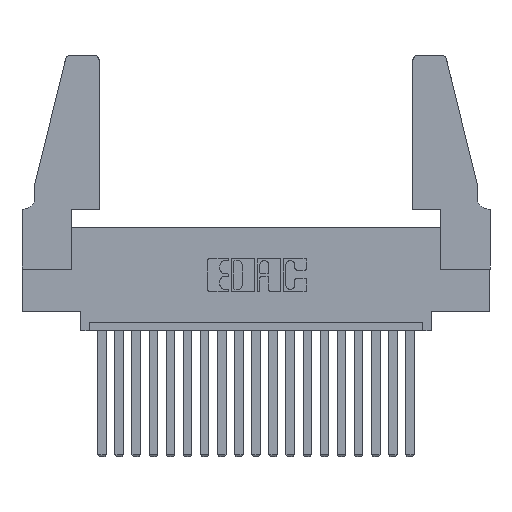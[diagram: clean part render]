
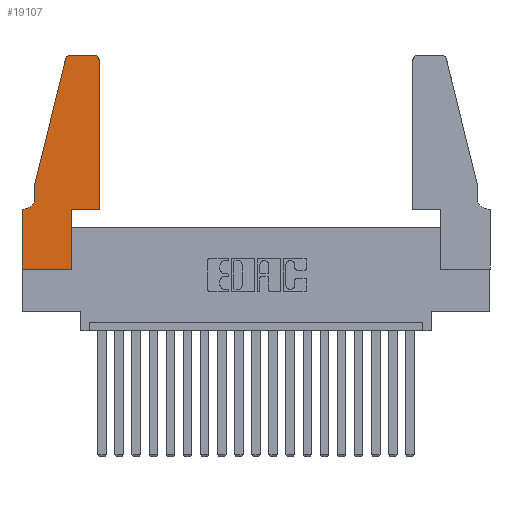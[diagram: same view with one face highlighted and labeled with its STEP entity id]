
A CAD part, top view. The second image highlights one B-rep face of the part: STEP entity #19107.
In plain terms, the highlighted planar face has unit normal (0, 0, 1).
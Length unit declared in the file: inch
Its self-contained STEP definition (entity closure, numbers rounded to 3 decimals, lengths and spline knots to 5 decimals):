
#226 = VERTEX_POINT ( 'NONE', #11601 ) ;
#607 = LINE ( 'NONE', #13470, #18976 ) ;
#1003 = FACE_OUTER_BOUND ( 'NONE', #8176, .T. ) ;
#1353 = EDGE_CURVE ( 'NONE', #18192, #9821, #18498, .T. ) ;
#1401 = EDGE_CURVE ( 'NONE', #15316, #226, #607, .T. ) ;
#1546 = CARTESIAN_POINT ( 'NONE',  ( 0.4505, 1.22, 0.37 ) ) ;
#1933 = EDGE_CURVE ( 'NONE', #9757, #9696, #8826, .T. ) ;
#2170 = DIRECTION ( 'NONE',  ( 1., 0., 0. ) ) ;
#2284 = VECTOR ( 'NONE', #16192, 39.37008 ) ;
#2330 = CARTESIAN_POINT ( 'NONE',  ( 0.4505, 0.35, 0.37 ) ) ;
#2348 = CARTESIAN_POINT ( 'NONE',  ( 0., 0., 0.37 ) ) ;
#2522 = ORIENTED_EDGE ( 'NONE', *, *, #6118, .T. ) ;
#2738 = CARTESIAN_POINT ( 'NONE',  ( 0.2605, 1.25, 0.37 ) ) ;
#2778 = LINE ( 'NONE', #10373, #2284 ) ;
#2810 = VERTEX_POINT ( 'NONE', #13792 ) ;
#2832 = DIRECTION ( 'NONE',  ( 0., -1., 0. ) ) ;
#3273 = VECTOR ( 'NONE', #3292, 39.37008 ) ;
#3292 = DIRECTION ( 'NONE',  ( 0., 1., 0. ) ) ;
#3576 = ORIENTED_EDGE ( 'NONE', *, *, #6120, .T. ) ;
#3849 = DIRECTION ( 'NONE',  ( 0., 1., 0. ) ) ;
#4026 = LINE ( 'NONE', #2738, #9886 ) ;
#4096 = ORIENTED_EDGE ( 'NONE', *, *, #1401, .T. ) ;
#4298 = DIRECTION ( 'NONE',  ( 0., 0., 1. ) ) ;
#4327 = LINE ( 'NONE', #17046, #19376 ) ;
#4695 = CARTESIAN_POINT ( 'NONE',  ( 0.2865, 0.35, 0.37 ) ) ;
#4701 = VECTOR ( 'NONE', #3849, 39.37008 ) ;
#4831 = AXIS2_PLACEMENT_3D ( 'NONE', #6130, #14998, #16462 ) ;
#5310 = ORIENTED_EDGE ( 'NONE', *, *, #9692, .T. ) ;
#5459 = DIRECTION ( 'NONE',  ( 0., -1., 0. ) ) ;
#5569 = CARTESIAN_POINT ( 'NONE',  ( 0.284, 1.25, 0.37 ) ) ;
#5737 = PLANE ( 'NONE',  #19244 ) ;
#5888 = CIRCLE ( 'NONE', #4831, 0.07 ) ;
#6118 = EDGE_CURVE ( 'NONE', #9821, #15316, #18614, .T. ) ;
#6120 = EDGE_CURVE ( 'NONE', #2810, #9757, #17877, .T. ) ;
#6130 = CARTESIAN_POINT ( 'NONE',  ( 0.0055, 0.42, 0.37 ) ) ;
#6135 = CARTESIAN_POINT ( 'NONE',  ( 0.284, 1.22, 0.37 ) ) ;
#6221 = DIRECTION ( 'NONE',  ( 1., 0., 0. ) ) ;
#6379 = VERTEX_POINT ( 'NONE', #4695 ) ;
#6643 = VERTEX_POINT ( 'NONE', #11308 ) ;
#6938 = ORIENTED_EDGE ( 'NONE', *, *, #11373, .T. ) ;
#7241 = DIRECTION ( 'NONE',  ( 1., 0., 0. ) ) ;
#7745 = VERTEX_POINT ( 'NONE', #16315 ) ;
#7936 = CARTESIAN_POINT ( 'NONE',  ( 0.2865, 0.35, 0.37 ) ) ;
#8176 = EDGE_LOOP ( 'NONE', ( #9922, #12229, #2522, #4096, #11889, #6938, #5310, #16405, #16954, #9813, #3576, #8730 ) ) ;
#8730 = ORIENTED_EDGE ( 'NONE', *, *, #1933, .T. ) ;
#8826 = CIRCLE ( 'NONE', #12240, 0.03 ) ;
#9294 = CARTESIAN_POINT ( 'NONE',  ( 0.4205, 1.22, 0.37 ) ) ;
#9692 = EDGE_CURVE ( 'NONE', #9926, #6643, #11031, .T. ) ;
#9696 = VERTEX_POINT ( 'NONE', #18745 ) ;
#9757 = VERTEX_POINT ( 'NONE', #1546 ) ;
#9813 = ORIENTED_EDGE ( 'NONE', *, *, #19306, .T. ) ;
#9821 = VERTEX_POINT ( 'NONE', #15637 ) ;
#9886 = VECTOR ( 'NONE', #18978, 39.37008 ) ;
#9922 = ORIENTED_EDGE ( 'NONE', *, *, #14367, .T. ) ;
#9926 = VERTEX_POINT ( 'NONE', #18589 ) ;
#10373 = CARTESIAN_POINT ( 'NONE',  ( 0.0755, 0.35, 0.37 ) ) ;
#10385 = DIRECTION ( 'NONE',  ( 0., 0., 1. ) ) ;
#11031 = LINE ( 'NONE', #2348, #17670 ) ;
#11308 = CARTESIAN_POINT ( 'NONE',  ( 0., 0., 0.37 ) ) ;
#11373 = EDGE_CURVE ( 'NONE', #7745, #9926, #2778, .T. ) ;
#11601 = CARTESIAN_POINT ( 'NONE',  ( 0.0755, 0.42, 0.37 ) ) ;
#11646 = VERTEX_POINT ( 'NONE', #19168 ) ;
#11889 = ORIENTED_EDGE ( 'NONE', *, *, #15219, .T. ) ;
#12181 = DIRECTION ( 'NONE',  ( 0., 0., 1. ) ) ;
#12229 = ORIENTED_EDGE ( 'NONE', *, *, #1353, .T. ) ;
#12240 = AXIS2_PLACEMENT_3D ( 'NONE', #9294, #12181, #6221 ) ;
#12658 = VECTOR ( 'NONE', #14824, 39.37008 ) ;
#13323 = CARTESIAN_POINT ( 'NONE',  ( 0., 0., 0.37 ) ) ;
#13470 = CARTESIAN_POINT ( 'NONE',  ( 0.0755, 0.5, 0.37 ) ) ;
#13792 = CARTESIAN_POINT ( 'NONE',  ( 0.4505, 0.35, 0.37 ) ) ;
#13854 = VECTOR ( 'NONE', #17701, 39.37008 ) ;
#14367 = EDGE_CURVE ( 'NONE', #9696, #18192, #4026, .T. ) ;
#14824 = DIRECTION ( 'NONE',  ( -0.239, -0.971, 0. ) ) ;
#14915 = AXIS2_PLACEMENT_3D ( 'NONE', #6135, #10385, #16583 ) ;
#14998 = DIRECTION ( 'NONE',  ( 0., 0., -1. ) ) ;
#15219 = EDGE_CURVE ( 'NONE', #226, #7745, #5888, .T. ) ;
#15272 = CARTESIAN_POINT ( 'NONE',  ( 0.0755, 0.5, 0.37 ) ) ;
#15316 = VERTEX_POINT ( 'NONE', #15272 ) ;
#15356 = EDGE_CURVE ( 'NONE', #11646, #6379, #17395, .T. ) ;
#15555 = EDGE_CURVE ( 'NONE', #6643, #11646, #17870, .T. ) ;
#15637 = CARTESIAN_POINT ( 'NONE',  ( 0.25487, 1.22718, 0.37 ) ) ;
#15898 = CARTESIAN_POINT ( 'NONE',  ( 0.0755, 0.5, 0.37 ) ) ;
#16192 = DIRECTION ( 'NONE',  ( -1., 0., 0. ) ) ;
#16263 = CARTESIAN_POINT ( 'NONE',  ( 0., 0.35, 0.37 ) ) ;
#16315 = CARTESIAN_POINT ( 'NONE',  ( 0.0055, 0.35, 0.37 ) ) ;
#16405 = ORIENTED_EDGE ( 'NONE', *, *, #15555, .T. ) ;
#16462 = DIRECTION ( 'NONE',  ( -1., 0., 0. ) ) ;
#16583 = DIRECTION ( 'NONE',  ( 1., 0., 0. ) ) ;
#16954 = ORIENTED_EDGE ( 'NONE', *, *, #15356, .T. ) ;
#17046 = CARTESIAN_POINT ( 'NONE',  ( 0.4505, 0.35, 0.37 ) ) ;
#17395 = LINE ( 'NONE', #7936, #3273 ) ;
#17670 = VECTOR ( 'NONE', #5459, 39.37008 ) ;
#17701 = DIRECTION ( 'NONE',  ( 1., 0., 0. ) ) ;
#17870 = LINE ( 'NONE', #13323, #13854 ) ;
#17877 = LINE ( 'NONE', #2330, #4701 ) ;
#18192 = VERTEX_POINT ( 'NONE', #5569 ) ;
#18498 = CIRCLE ( 'NONE', #14915, 0.03 ) ;
#18589 = CARTESIAN_POINT ( 'NONE',  ( 0., 0.35, 0.37 ) ) ;
#18614 = LINE ( 'NONE', #15898, #12658 ) ;
#18745 = CARTESIAN_POINT ( 'NONE',  ( 0.4205, 1.25, 0.37 ) ) ;
#18976 = VECTOR ( 'NONE', #2832, 39.37008 ) ;
#18978 = DIRECTION ( 'NONE',  ( -1., 0., 0. ) ) ;
#19107 = ADVANCED_FACE ( 'NONE', ( #1003 ), #5737, .T. ) ;
#19168 = CARTESIAN_POINT ( 'NONE',  ( 0.2865, 0., 0.37 ) ) ;
#19244 = AXIS2_PLACEMENT_3D ( 'NONE', #16263, #4298, #7241 ) ;
#19306 = EDGE_CURVE ( 'NONE', #6379, #2810, #4327, .T. ) ;
#19376 = VECTOR ( 'NONE', #2170, 39.37008 ) ;
